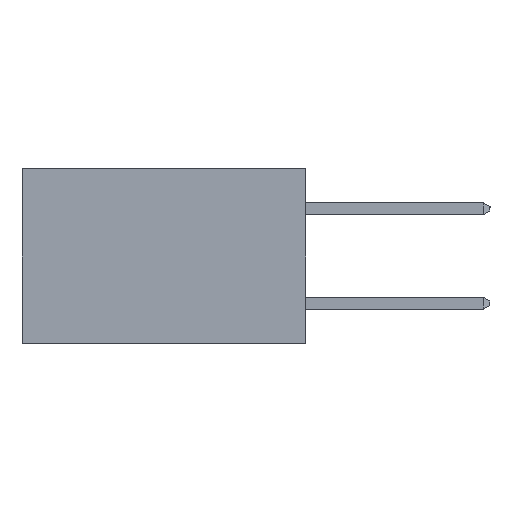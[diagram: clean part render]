
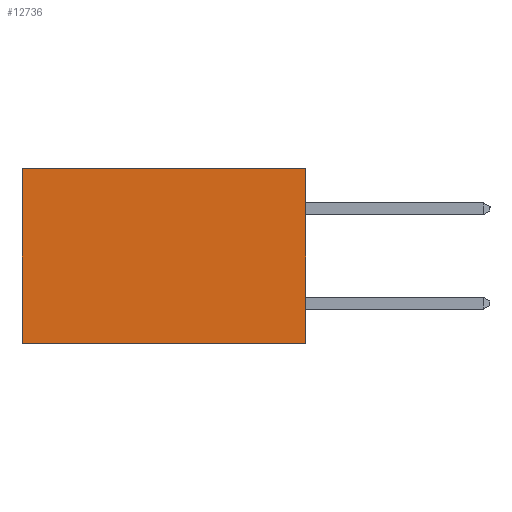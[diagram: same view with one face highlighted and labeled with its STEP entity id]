
A CAD part, left-side view. The second image highlights one B-rep face of the part: STEP entity #12736.
In plain terms, the highlighted planar face has unit normal (-1, 0, 0).
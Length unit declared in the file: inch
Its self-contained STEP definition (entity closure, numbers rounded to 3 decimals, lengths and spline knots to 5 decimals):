
#367 = EDGE_CURVE ( 'NONE', #16790, #807, #7822, .T. ) ;
#807 = VERTEX_POINT ( 'NONE', #15003 ) ;
#1184 = DIRECTION ( 'NONE',  ( 0., 0., -1. ) ) ;
#1222 = DIRECTION ( 'NONE',  ( 0., 0., -1. ) ) ;
#2701 = VECTOR ( 'NONE', #16728, 39.37008 ) ;
#3121 = PLANE ( 'NONE',  #14130 ) ;
#3548 = ORIENTED_EDGE ( 'NONE', *, *, #3669, .F. ) ;
#3669 = EDGE_CURVE ( 'NONE', #10505, #807, #10401, .T. ) ;
#5005 = VERTEX_POINT ( 'NONE', #17853 ) ;
#5353 = ORIENTED_EDGE ( 'NONE', *, *, #10257, .F. ) ;
#5459 = CARTESIAN_POINT ( 'NONE',  ( 0.2615, 0., -0.37 ) ) ;
#7822 = LINE ( 'NONE', #17596, #9511 ) ;
#8605 = CARTESIAN_POINT ( 'NONE',  ( 0.2615, 0., -0.37 ) ) ;
#9035 = CARTESIAN_POINT ( 'NONE',  ( 0.2615, 0., -0.37 ) ) ;
#9511 = VECTOR ( 'NONE', #10661, 39.37008 ) ;
#10257 = EDGE_CURVE ( 'NONE', #5005, #10505, #16361, .T. ) ;
#10401 = LINE ( 'NONE', #15121, #14852 ) ;
#10493 = DIRECTION ( 'NONE',  ( 0., 1., 0. ) ) ;
#10505 = VERTEX_POINT ( 'NONE', #9035 ) ;
#10661 = DIRECTION ( 'NONE',  ( 0., 0., -1. ) ) ;
#11455 = ORIENTED_EDGE ( 'NONE', *, *, #11657, .T. ) ;
#11657 = EDGE_CURVE ( 'NONE', #5005, #16790, #16365, .T. ) ;
#12022 = VECTOR ( 'NONE', #1184, 39.37008 ) ;
#12534 = CARTESIAN_POINT ( 'NONE',  ( 0.2615, 0., 0. ) ) ;
#12736 = ADVANCED_FACE ( 'NONE', ( #15641 ), #3121, .F. ) ;
#14063 = EDGE_LOOP ( 'NONE', ( #17646, #3548, #5353, #11455 ) ) ;
#14130 = AXIS2_PLACEMENT_3D ( 'NONE', #8605, #17935, #1222 ) ;
#14852 = VECTOR ( 'NONE', #10493, 39.37008 ) ;
#15003 = CARTESIAN_POINT ( 'NONE',  ( 0.2615, 0.6, -0.37 ) ) ;
#15121 = CARTESIAN_POINT ( 'NONE',  ( 0.2615, 0., -0.37 ) ) ;
#15641 = FACE_OUTER_BOUND ( 'NONE', #14063, .T. ) ;
#16361 = LINE ( 'NONE', #5459, #12022 ) ;
#16365 = LINE ( 'NONE', #12534, #2701 ) ;
#16728 = DIRECTION ( 'NONE',  ( 0., 1., 0. ) ) ;
#16790 = VERTEX_POINT ( 'NONE', #17607 ) ;
#17596 = CARTESIAN_POINT ( 'NONE',  ( 0.2615, 0.6, -0.37 ) ) ;
#17607 = CARTESIAN_POINT ( 'NONE',  ( 0.2615, 0.6, 0. ) ) ;
#17646 = ORIENTED_EDGE ( 'NONE', *, *, #367, .T. ) ;
#17853 = CARTESIAN_POINT ( 'NONE',  ( 0.2615, 0., 0. ) ) ;
#17935 = DIRECTION ( 'NONE',  ( 1., 0., 0. ) ) ;
